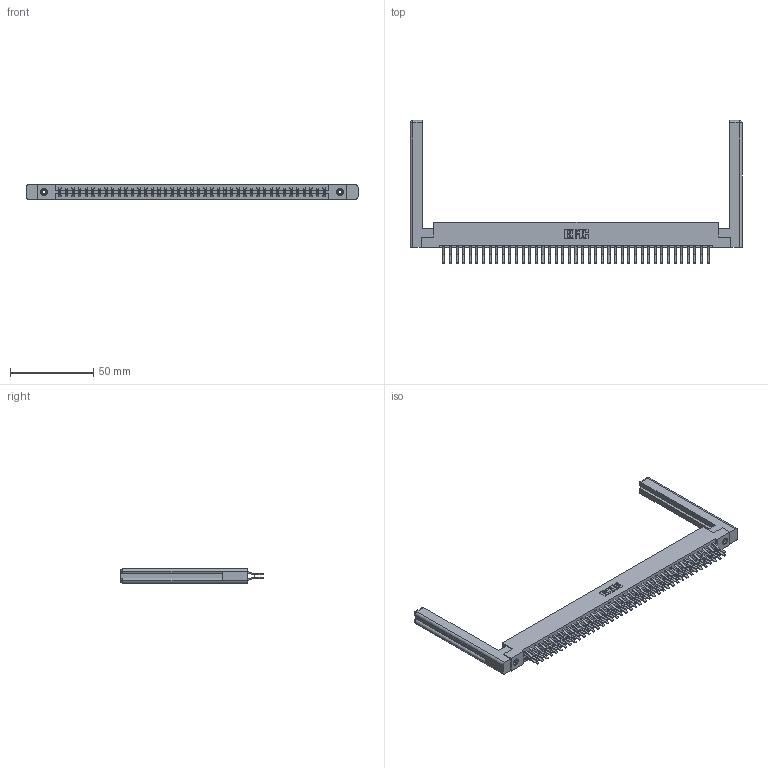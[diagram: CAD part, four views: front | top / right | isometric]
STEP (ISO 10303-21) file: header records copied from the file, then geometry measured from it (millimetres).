
FILE_DESCRIPTION (( 'STEP AP203' ), '1' );
FILE_NAME ('387-082-560-258.STEP', '2019-10-23T00:39:37', ( '' ), ( '' ), 'SwSTEP 2.0', 'SolidWorks 2016', '' );
FILE_SCHEMA (( 'CONFIG_CONTROL_DESIGN' ));
Length unit declared in the file: inch
Products named in the file (5): 345-250-001_345-250-001-102; 345-292-001_560 Tail; 337 Part_Flush Mounting Lugs - 0.156 Dia-TI; 307-220-058; 387-082-560-258
Assembly tree (87 placements, depth 2):
  387-082-560-258
    337 Part_Flush Mounting Lugs - 0.156 Dia-TI
    345-292-001_560 Tail  x82
    345-250-001_345-250-001-102  x2
    307-220-058  x2
Bounding box: 199.09 x 85.87 x 9.4 mm (x, y, z)
Volume: 28647.7 mm3; surface area: 30904.5 mm2
Topology: 87 solids, 87 shells, 4848 faces, 14359 edges, 9450 vertices
Faces by surface type: plane 3270, cylinder 1554, cone 12, torus 12
Entity records: 34640 total; most frequent: CARTESIAN_POINT 5845, ORIENTED_EDGE 5720, DIRECTION 4992, EDGE_CURVE 2860, LINE 2680, VECTOR 2680, VERTEX_POINT 1898, AXIS2_PLACEMENT_3D 1156
